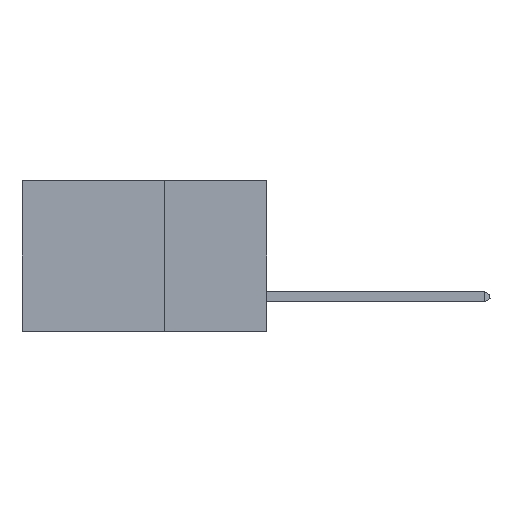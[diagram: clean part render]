
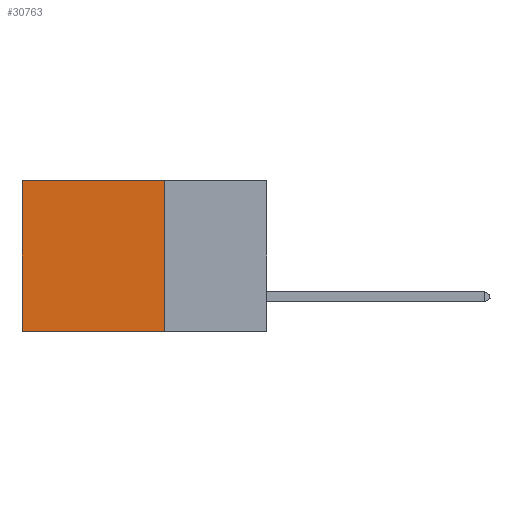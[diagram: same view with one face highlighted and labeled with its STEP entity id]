
A CAD part, left-side view. The second image highlights one B-rep face of the part: STEP entity #30763.
In plain terms, the highlighted planar face has unit normal (-1, 0, 0).
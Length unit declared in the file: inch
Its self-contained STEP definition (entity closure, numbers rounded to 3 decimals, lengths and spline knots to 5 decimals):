
#1222 = DIRECTION ( 'NONE',  ( 0., 1., 0. ) ) ;
#1781 = DIRECTION ( 'NONE',  ( 0., 1., 0. ) ) ;
#2584 = FACE_OUTER_BOUND ( 'NONE', #31354, .T. ) ;
#4141 = ORIENTED_EDGE ( 'NONE', *, *, #18048, .T. ) ;
#4370 = AXIS2_PLACEMENT_3D ( 'NONE', #27860, #38373, #18025 ) ;
#6574 = CARTESIAN_POINT ( 'NONE',  ( 0.2875, 0.25, -0.37 ) ) ;
#7481 = VERTEX_POINT ( 'NONE', #26785 ) ;
#7996 = CARTESIAN_POINT ( 'NONE',  ( 0.2875, 0.25, 0. ) ) ;
#8224 = VERTEX_POINT ( 'NONE', #29817 ) ;
#8331 = ORIENTED_EDGE ( 'NONE', *, *, #16414, .F. ) ;
#11294 = EDGE_CURVE ( 'NONE', #37702, #7481, #36943, .T. ) ;
#11813 = CARTESIAN_POINT ( 'NONE',  ( 0.2875, 0.25, 0. ) ) ;
#15046 = ORIENTED_EDGE ( 'NONE', *, *, #30538, .F. ) ;
#16307 = ORIENTED_EDGE ( 'NONE', *, *, #11294, .T. ) ;
#16414 = EDGE_CURVE ( 'NONE', #36939, #8224, #42708, .T. ) ;
#18025 = DIRECTION ( 'NONE',  ( 0., 0., -1. ) ) ;
#18048 = EDGE_CURVE ( 'NONE', #7481, #8224, #37766, .T. ) ;
#18228 = DIRECTION ( 'NONE',  ( 0., 0., -1. ) ) ;
#19399 = VECTOR ( 'NONE', #18228, 39.37008 ) ;
#20047 = VECTOR ( 'NONE', #31913, 39.37008 ) ;
#21341 = CARTESIAN_POINT ( 'NONE',  ( 0.2875, 0.25, -0.37 ) ) ;
#21396 = PLANE ( 'NONE',  #4370 ) ;
#26785 = CARTESIAN_POINT ( 'NONE',  ( 0.2875, 0.6, 0. ) ) ;
#27860 = CARTESIAN_POINT ( 'NONE',  ( 0.2875, 0.25, 0. ) ) ;
#28577 = VECTOR ( 'NONE', #1781, 39.37008 ) ;
#29817 = CARTESIAN_POINT ( 'NONE',  ( 0.2875, 0.6, -0.37 ) ) ;
#30538 = EDGE_CURVE ( 'NONE', #37702, #36939, #35647, .T. ) ;
#30763 = ADVANCED_FACE ( 'NONE', ( #2584 ), #21396, .F. ) ;
#31128 = CARTESIAN_POINT ( 'NONE',  ( 0.2875, 0.25, 0. ) ) ;
#31354 = EDGE_LOOP ( 'NONE', ( #4141, #8331, #15046, #16307 ) ) ;
#31461 = CARTESIAN_POINT ( 'NONE',  ( 0.2875, 0.6, 0. ) ) ;
#31913 = DIRECTION ( 'NONE',  ( 0., 0., -1. ) ) ;
#35647 = LINE ( 'NONE', #7996, #19399 ) ;
#36939 = VERTEX_POINT ( 'NONE', #6574 ) ;
#36943 = LINE ( 'NONE', #11813, #28577 ) ;
#37702 = VERTEX_POINT ( 'NONE', #31128 ) ;
#37766 = LINE ( 'NONE', #31461, #20047 ) ;
#38373 = DIRECTION ( 'NONE',  ( 1., 0., 0. ) ) ;
#42708 = LINE ( 'NONE', #21341, #43232 ) ;
#43232 = VECTOR ( 'NONE', #1222, 39.37008 ) ;
